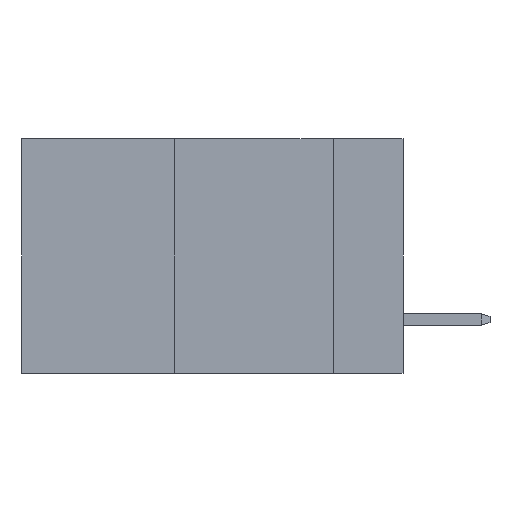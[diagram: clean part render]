
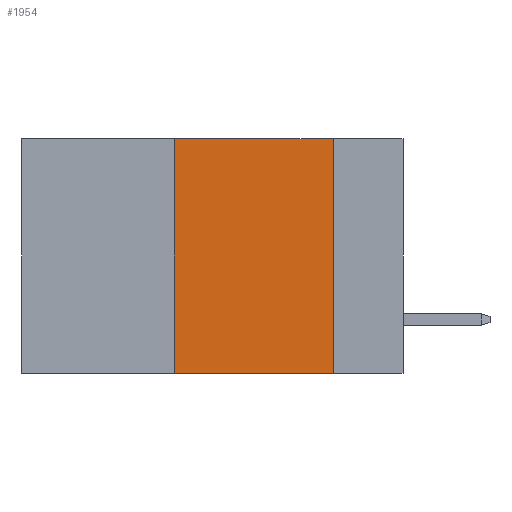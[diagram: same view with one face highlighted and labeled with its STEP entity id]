
A CAD part, left-side view. The second image highlights one B-rep face of the part: STEP entity #1954.
In plain terms, the highlighted planar face has unit normal (-1, 0, 0).
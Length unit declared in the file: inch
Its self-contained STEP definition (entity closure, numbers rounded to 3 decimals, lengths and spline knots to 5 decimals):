
#123 = ORIENTED_EDGE ( 'NONE', *, *, #3679, .F. ) ;
#326 = EDGE_LOOP ( 'NONE', ( #6140, #5067, #123, #3780 ) ) ;
#532 = VERTEX_POINT ( 'NONE', #3312 ) ;
#572 = EDGE_CURVE ( 'NONE', #10585, #532, #6630, .T. ) ;
#768 = VECTOR ( 'NONE', #3389, 39.37008 ) ;
#973 = DIRECTION ( 'NONE',  ( 1., 0., 0. ) ) ;
#1426 = CARTESIAN_POINT ( 'NONE',  ( 0., 0.11, 0. ) ) ;
#1797 = CARTESIAN_POINT ( 'NONE',  ( 0., 0.6, 0. ) ) ;
#1854 = VECTOR ( 'NONE', #7011, 39.37008 ) ;
#1879 = LINE ( 'NONE', #7730, #1854 ) ;
#1916 = EDGE_CURVE ( 'NONE', #10290, #532, #3554, .T. ) ;
#1954 = ADVANCED_FACE ( 'NONE', ( #8419 ), #9294, .F. ) ;
#2431 = CARTESIAN_POINT ( 'NONE',  ( 0., 0.11, 0. ) ) ;
#2783 = DIRECTION ( 'NONE',  ( 0., 0., -1. ) ) ;
#3312 = CARTESIAN_POINT ( 'NONE',  ( 0., 0.11, -0.37 ) ) ;
#3389 = DIRECTION ( 'NONE',  ( 0., -1., 0. ) ) ;
#3554 = LINE ( 'NONE', #6879, #768 ) ;
#3578 = AXIS2_PLACEMENT_3D ( 'NONE', #1797, #973, #2783 ) ;
#3610 = CARTESIAN_POINT ( 'NONE',  ( 0., 0.36, 0. ) ) ;
#3679 = EDGE_CURVE ( 'NONE', #10290, #4539, #1879, .T. ) ;
#3780 = ORIENTED_EDGE ( 'NONE', *, *, #1916, .T. ) ;
#4539 = VERTEX_POINT ( 'NONE', #3610 ) ;
#4632 = CARTESIAN_POINT ( 'NONE',  ( 0., 0.6, 0. ) ) ;
#5067 = ORIENTED_EDGE ( 'NONE', *, *, #7102, .F. ) ;
#5558 = LINE ( 'NONE', #4632, #7110 ) ;
#6140 = ORIENTED_EDGE ( 'NONE', *, *, #572, .F. ) ;
#6630 = LINE ( 'NONE', #2431, #9114 ) ;
#6679 = CARTESIAN_POINT ( 'NONE',  ( 0., 0.36, -0.37 ) ) ;
#6879 = CARTESIAN_POINT ( 'NONE',  ( 0., 0.6, -0.37 ) ) ;
#7011 = DIRECTION ( 'NONE',  ( 0., 0., 1. ) ) ;
#7102 = EDGE_CURVE ( 'NONE', #4539, #10585, #5558, .T. ) ;
#7110 = VECTOR ( 'NONE', #7303, 39.37008 ) ;
#7303 = DIRECTION ( 'NONE',  ( 0., -1., 0. ) ) ;
#7730 = CARTESIAN_POINT ( 'NONE',  ( 0., 0.36, 0. ) ) ;
#8419 = FACE_OUTER_BOUND ( 'NONE', #326, .T. ) ;
#9114 = VECTOR ( 'NONE', #10748, 39.37008 ) ;
#9294 = PLANE ( 'NONE',  #3578 ) ;
#10290 = VERTEX_POINT ( 'NONE', #6679 ) ;
#10585 = VERTEX_POINT ( 'NONE', #1426 ) ;
#10748 = DIRECTION ( 'NONE',  ( 0., 0., -1. ) ) ;
